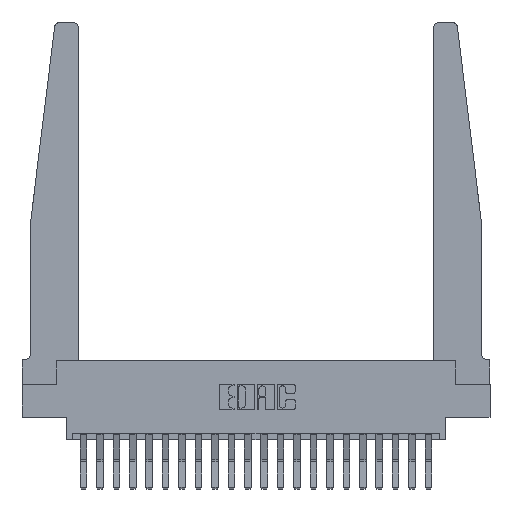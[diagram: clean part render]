
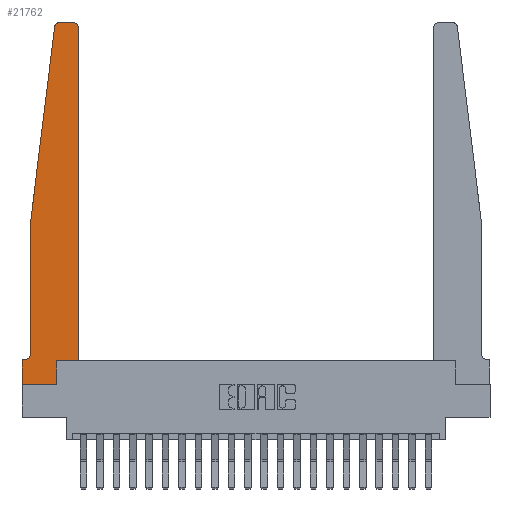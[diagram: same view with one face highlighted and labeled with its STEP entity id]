
A CAD part, top view. The second image highlights one B-rep face of the part: STEP entity #21762.
In plain terms, the highlighted planar face has unit normal (0, 0, 1).
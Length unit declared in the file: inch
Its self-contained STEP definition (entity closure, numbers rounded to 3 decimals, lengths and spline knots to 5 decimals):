
#70 = DIRECTION ( 'NONE',  ( 0., 0., 1. ) ) ;
#78 = CARTESIAN_POINT ( 'NONE',  ( 0., 0., 0.37 ) ) ;
#157 = ORIENTED_EDGE ( 'NONE', *, *, #15314, .T. ) ;
#342 = DIRECTION ( 'NONE',  ( 0., -1., 0. ) ) ;
#481 = DIRECTION ( 'NONE',  ( 1., 0., 0. ) ) ;
#578 = CARTESIAN_POINT ( 'NONE',  ( 0., 0., 0.37 ) ) ;
#722 = DIRECTION ( 'NONE',  ( 1., 0., 0. ) ) ;
#972 = CARTESIAN_POINT ( 'NONE',  ( 0., 0., 0.37 ) ) ;
#977 = EDGE_LOOP ( 'NONE', ( #12799, #15851, #3144, #8119, #17768, #14927, #157, #20497, #10141, #7756, #17100, #14938 ) ) ;
#1153 = AXIS2_PLACEMENT_3D ( 'NONE', #20883, #10733, #481 ) ;
#1599 = LINE ( 'NONE', #10608, #14116 ) ;
#2270 = LINE ( 'NONE', #10757, #13724 ) ;
#2538 = VERTEX_POINT ( 'NONE', #7460 ) ;
#2742 = CARTESIAN_POINT ( 'NONE',  ( 0.065, 1.25, 0.37 ) ) ;
#3112 = EDGE_CURVE ( 'NONE', #13183, #10576, #5933, .T. ) ;
#3144 = ORIENTED_EDGE ( 'NONE', *, *, #9943, .T. ) ;
#3710 = EDGE_CURVE ( 'NONE', #17141, #5604, #4295, .T. ) ;
#3772 = CARTESIAN_POINT ( 'NONE',  ( 0.065, 0.2375, 0.37 ) ) ;
#3776 = EDGE_CURVE ( 'NONE', #10576, #15177, #16779, .T. ) ;
#4008 = DIRECTION ( 'NONE',  ( -1., 0., 0. ) ) ;
#4044 = DIRECTION ( 'NONE',  ( 0., -1., 0. ) ) ;
#4187 = VECTOR ( 'NONE', #9619, 39.37008 ) ;
#4295 = CIRCLE ( 'NONE', #1153, 0.03 ) ;
#4333 = CARTESIAN_POINT ( 'NONE',  ( 0.24675, 2.72367, 0.37 ) ) ;
#4341 = AXIS2_PLACEMENT_3D ( 'NONE', #5945, #17798, #7652 ) ;
#4420 = EDGE_CURVE ( 'NONE', #18690, #6584, #9931, .T. ) ;
#5149 = CIRCLE ( 'NONE', #9014, 0.03 ) ;
#5225 = VERTEX_POINT ( 'NONE', #4333 ) ;
#5371 = VECTOR ( 'NONE', #10638, 39.37008 ) ;
#5604 = VERTEX_POINT ( 'NONE', #12062 ) ;
#5933 = CIRCLE ( 'NONE', #4341, 0.05 ) ;
#5945 = CARTESIAN_POINT ( 'NONE',  ( 0.015, 0.2375, 0.37 ) ) ;
#6027 = LINE ( 'NONE', #2742, #10052 ) ;
#6584 = VERTEX_POINT ( 'NONE', #9007 ) ;
#6786 = EDGE_CURVE ( 'NONE', #15116, #15840, #8742, .T. ) ;
#6841 = FACE_OUTER_BOUND ( 'NONE', #977, .T. ) ;
#7460 = CARTESIAN_POINT ( 'NONE',  ( 0.27653, 2.75, 0.37 ) ) ;
#7652 = DIRECTION ( 'NONE',  ( -1., 0., 0. ) ) ;
#7756 = ORIENTED_EDGE ( 'NONE', *, *, #4420, .T. ) ;
#8119 = ORIENTED_EDGE ( 'NONE', *, *, #12409, .T. ) ;
#8550 = AXIS2_PLACEMENT_3D ( 'NONE', #10353, #70, #12020 ) ;
#8623 = PLANE ( 'NONE',  #8550 ) ;
#8742 = LINE ( 'NONE', #972, #4187 ) ;
#8746 = VECTOR ( 'NONE', #10921, 39.37008 ) ;
#8826 = EDGE_CURVE ( 'NONE', #5604, #2538, #12692, .T. ) ;
#9007 = CARTESIAN_POINT ( 'NONE',  ( 0.425, 0.18, 0.37 ) ) ;
#9014 = AXIS2_PLACEMENT_3D ( 'NONE', #21132, #10980, #722 ) ;
#9619 = DIRECTION ( 'NONE',  ( 1., 0., 0. ) ) ;
#9753 = EDGE_CURVE ( 'NONE', #6584, #17141, #2270, .T. ) ;
#9931 = LINE ( 'NONE', #20786, #5371 ) ;
#9943 = EDGE_CURVE ( 'NONE', #5225, #14837, #6027, .T. ) ;
#10052 = VECTOR ( 'NONE', #14632, 39.37008 ) ;
#10141 = ORIENTED_EDGE ( 'NONE', *, *, #14142, .T. ) ;
#10353 = CARTESIAN_POINT ( 'NONE',  ( 0., 0.1875, 0.37 ) ) ;
#10576 = VERTEX_POINT ( 'NONE', #21911 ) ;
#10608 = CARTESIAN_POINT ( 'NONE',  ( 0.065, 1.25, 0.37 ) ) ;
#10638 = DIRECTION ( 'NONE',  ( 1., 0., 0. ) ) ;
#10733 = DIRECTION ( 'NONE',  ( 0., 0., 1. ) ) ;
#10757 = CARTESIAN_POINT ( 'NONE',  ( 0.425, 0.18, 0.37 ) ) ;
#10808 = CARTESIAN_POINT ( 'NONE',  ( 0.065, 0.1875, 0.37 ) ) ;
#10921 = DIRECTION ( 'NONE',  ( -1., 0., 0. ) ) ;
#10980 = DIRECTION ( 'NONE',  ( 0., 0., 1. ) ) ;
#11594 = EDGE_CURVE ( 'NONE', #2538, #5225, #5149, .T. ) ;
#12020 = DIRECTION ( 'NONE',  ( 1., 0., 0. ) ) ;
#12062 = CARTESIAN_POINT ( 'NONE',  ( 0.395, 2.75, 0.37 ) ) ;
#12409 = EDGE_CURVE ( 'NONE', #14837, #13183, #1599, .T. ) ;
#12593 = CARTESIAN_POINT ( 'NONE',  ( 0.25, 2.75, 0.37 ) ) ;
#12637 = CARTESIAN_POINT ( 'NONE',  ( 0.2605, 0.18, 0.37 ) ) ;
#12692 = LINE ( 'NONE', #12593, #8746 ) ;
#12799 = ORIENTED_EDGE ( 'NONE', *, *, #8826, .T. ) ;
#13008 = VECTOR ( 'NONE', #21854, 39.37008 ) ;
#13183 = VERTEX_POINT ( 'NONE', #3772 ) ;
#13724 = VECTOR ( 'NONE', #19190, 39.37008 ) ;
#13761 = CARTESIAN_POINT ( 'NONE',  ( 0.2605, 0., 0.37 ) ) ;
#14116 = VECTOR ( 'NONE', #342, 39.37008 ) ;
#14142 = EDGE_CURVE ( 'NONE', #15840, #18690, #17536, .T. ) ;
#14632 = DIRECTION ( 'NONE',  ( -0.122, -0.992, 0. ) ) ;
#14837 = VERTEX_POINT ( 'NONE', #15055 ) ;
#14927 = ORIENTED_EDGE ( 'NONE', *, *, #3776, .T. ) ;
#14938 = ORIENTED_EDGE ( 'NONE', *, *, #3710, .T. ) ;
#15055 = CARTESIAN_POINT ( 'NONE',  ( 0.065, 1.25, 0.37 ) ) ;
#15116 = VERTEX_POINT ( 'NONE', #78 ) ;
#15177 = VERTEX_POINT ( 'NONE', #20697 ) ;
#15314 = EDGE_CURVE ( 'NONE', #15177, #15116, #20110, .T. ) ;
#15577 = VECTOR ( 'NONE', #4044, 39.37008 ) ;
#15840 = VERTEX_POINT ( 'NONE', #13761 ) ;
#15851 = ORIENTED_EDGE ( 'NONE', *, *, #11594, .T. ) ;
#16779 = LINE ( 'NONE', #10808, #21077 ) ;
#17100 = ORIENTED_EDGE ( 'NONE', *, *, #9753, .T. ) ;
#17141 = VERTEX_POINT ( 'NONE', #18617 ) ;
#17536 = LINE ( 'NONE', #20151, #13008 ) ;
#17768 = ORIENTED_EDGE ( 'NONE', *, *, #3112, .T. ) ;
#17798 = DIRECTION ( 'NONE',  ( 0., 0., -1. ) ) ;
#18617 = CARTESIAN_POINT ( 'NONE',  ( 0.425, 2.72, 0.37 ) ) ;
#18690 = VERTEX_POINT ( 'NONE', #12637 ) ;
#19190 = DIRECTION ( 'NONE',  ( 0., 1., 0. ) ) ;
#20110 = LINE ( 'NONE', #578, #15577 ) ;
#20151 = CARTESIAN_POINT ( 'NONE',  ( 0.2605, 0.18, 0.37 ) ) ;
#20497 = ORIENTED_EDGE ( 'NONE', *, *, #6786, .T. ) ;
#20697 = CARTESIAN_POINT ( 'NONE',  ( 0., 0.1875, 0.37 ) ) ;
#20786 = CARTESIAN_POINT ( 'NONE',  ( 0.425, 0.18, 0.37 ) ) ;
#20883 = CARTESIAN_POINT ( 'NONE',  ( 0.395, 2.72, 0.37 ) ) ;
#21077 = VECTOR ( 'NONE', #4008, 39.37008 ) ;
#21132 = CARTESIAN_POINT ( 'NONE',  ( 0.27653, 2.72, 0.37 ) ) ;
#21762 = ADVANCED_FACE ( 'NONE', ( #6841 ), #8623, .T. ) ;
#21854 = DIRECTION ( 'NONE',  ( 0., 1., 0. ) ) ;
#21911 = CARTESIAN_POINT ( 'NONE',  ( 0.015, 0.1875, 0.37 ) ) ;
